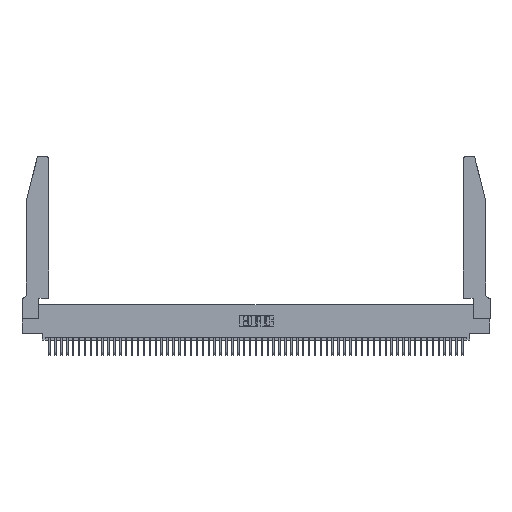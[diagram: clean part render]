
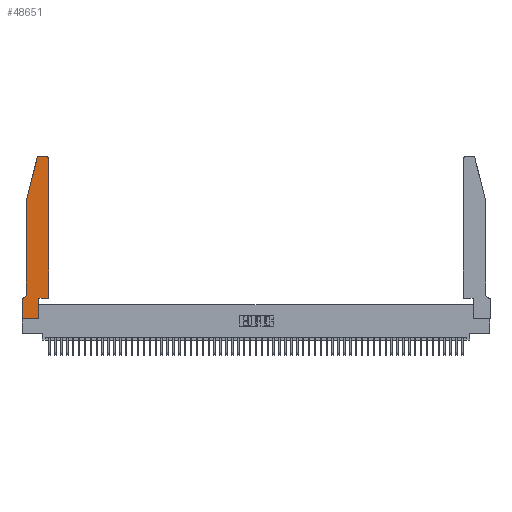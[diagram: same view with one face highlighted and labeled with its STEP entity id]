
A CAD part, top view. The second image highlights one B-rep face of the part: STEP entity #48651.
In plain terms, the highlighted planar face has unit normal (0, 0, 1).
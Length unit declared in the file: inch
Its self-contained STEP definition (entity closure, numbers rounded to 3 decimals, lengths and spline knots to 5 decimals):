
#319 = CARTESIAN_POINT ( 'NONE',  ( 0.0755, 2., 0.37 ) ) ;
#445 = AXIS2_PLACEMENT_3D ( 'NONE', #43484, #18274, #47694 ) ;
#1582 = EDGE_CURVE ( 'NONE', #11955, #36838, #24573, .T. ) ;
#1751 = CARTESIAN_POINT ( 'NONE',  ( 0.0055, 0.42, 0.37 ) ) ;
#1983 = CARTESIAN_POINT ( 'NONE',  ( 0., 0.35, 0.37 ) ) ;
#2160 = VECTOR ( 'NONE', #12118, 39.37008 ) ;
#3042 = CARTESIAN_POINT ( 'NONE',  ( 0.284, 2.75, 0.37 ) ) ;
#3897 = ORIENTED_EDGE ( 'NONE', *, *, #4796, .T. ) ;
#4695 = EDGE_CURVE ( 'NONE', #5324, #38068, #33540, .T. ) ;
#4796 = EDGE_CURVE ( 'NONE', #36075, #14396, #26893, .T. ) ;
#5324 = VERTEX_POINT ( 'NONE', #27573 ) ;
#6003 = DIRECTION ( 'NONE',  ( -1., 0., 0. ) ) ;
#6811 = ORIENTED_EDGE ( 'NONE', *, *, #1582, .T. ) ;
#7475 = CARTESIAN_POINT ( 'NONE',  ( 0.2865, 0.35, 0.37 ) ) ;
#7748 = EDGE_CURVE ( 'NONE', #14396, #22877, #35192, .T. ) ;
#8241 = EDGE_CURVE ( 'NONE', #36838, #21234, #42380, .T. ) ;
#8621 = VECTOR ( 'NONE', #40121, 39.37008 ) ;
#8830 = DIRECTION ( 'NONE',  ( 1., 0., 0. ) ) ;
#9283 = DIRECTION ( 'NONE',  ( -1., 0., 0. ) ) ;
#9639 = CARTESIAN_POINT ( 'NONE',  ( 0.2865, 0.35, 0.37 ) ) ;
#10487 = DIRECTION ( 'NONE',  ( 0., 0., 1. ) ) ;
#10995 = EDGE_CURVE ( 'NONE', #21234, #36075, #44745, .T. ) ;
#11955 = VERTEX_POINT ( 'NONE', #27336 ) ;
#12118 = DIRECTION ( 'NONE',  ( 0., -1., 0. ) ) ;
#13052 = CARTESIAN_POINT ( 'NONE',  ( 0.4505, 0.35, 0.37 ) ) ;
#14396 = VERTEX_POINT ( 'NONE', #27456 ) ;
#15655 = CARTESIAN_POINT ( 'NONE',  ( 0., 0., 0.37 ) ) ;
#16152 = VECTOR ( 'NONE', #9283, 39.37008 ) ;
#16214 = CARTESIAN_POINT ( 'NONE',  ( 0., 0., 0.37 ) ) ;
#17419 = ORIENTED_EDGE ( 'NONE', *, *, #7748, .T. ) ;
#18274 = DIRECTION ( 'NONE',  ( 0., 0., 1. ) ) ;
#18337 = VECTOR ( 'NONE', #19895, 39.37008 ) ;
#18453 = ORIENTED_EDGE ( 'NONE', *, *, #51909, .T. ) ;
#18457 = EDGE_CURVE ( 'NONE', #36590, #21401, #35798, .T. ) ;
#18555 = ORIENTED_EDGE ( 'NONE', *, *, #10995, .T. ) ;
#19895 = DIRECTION ( 'NONE',  ( 0., 1., 0. ) ) ;
#20871 = CARTESIAN_POINT ( 'NONE',  ( 0.0755, 0.42, 0.37 ) ) ;
#21234 = VERTEX_POINT ( 'NONE', #7475 ) ;
#21401 = VERTEX_POINT ( 'NONE', #20871 ) ;
#21773 = CARTESIAN_POINT ( 'NONE',  ( 0.2605, 2.75, 0.37 ) ) ;
#22257 = CIRCLE ( 'NONE', #445, 0.03 ) ;
#22319 = VECTOR ( 'NONE', #8830, 39.37008 ) ;
#22877 = VERTEX_POINT ( 'NONE', #31400 ) ;
#23267 = DIRECTION ( 'NONE',  ( 0., 0., 1. ) ) ;
#24428 = CIRCLE ( 'NONE', #27791, 0.07 ) ;
#24573 = LINE ( 'NONE', #16214, #49570 ) ;
#26893 = LINE ( 'NONE', #36698, #18337 ) ;
#27336 = CARTESIAN_POINT ( 'NONE',  ( 0., 0., 0.37 ) ) ;
#27456 = CARTESIAN_POINT ( 'NONE',  ( 0.4505, 2.72, 0.37 ) ) ;
#27573 = CARTESIAN_POINT ( 'NONE',  ( 0.0055, 0.35, 0.37 ) ) ;
#27791 = AXIS2_PLACEMENT_3D ( 'NONE', #1751, #31198, #6003 ) ;
#27898 = EDGE_CURVE ( 'NONE', #38068, #11955, #40880, .T. ) ;
#28631 = ORIENTED_EDGE ( 'NONE', *, *, #18457, .T. ) ;
#30777 = ORIENTED_EDGE ( 'NONE', *, *, #34444, .T. ) ;
#31198 = DIRECTION ( 'NONE',  ( 0., 0., -1. ) ) ;
#31400 = CARTESIAN_POINT ( 'NONE',  ( 0.4205, 2.75, 0.37 ) ) ;
#32064 = CARTESIAN_POINT ( 'NONE',  ( 0.0755, 0.35, 0.37 ) ) ;
#32835 = VERTEX_POINT ( 'NONE', #3042 ) ;
#33135 = CARTESIAN_POINT ( 'NONE',  ( 0.0755, 2., 0.37 ) ) ;
#33389 = ORIENTED_EDGE ( 'NONE', *, *, #49788, .T. ) ;
#33540 = LINE ( 'NONE', #32064, #51865 ) ;
#33965 = AXIS2_PLACEMENT_3D ( 'NONE', #48462, #23267, #52670 ) ;
#34058 = DIRECTION ( 'NONE',  ( -0.239, -0.971, 0. ) ) ;
#34444 = EDGE_CURVE ( 'NONE', #21401, #5324, #24428, .T. ) ;
#35192 = CIRCLE ( 'NONE', #33965, 0.03 ) ;
#35705 = CARTESIAN_POINT ( 'NONE',  ( 0.0755, 2., 0.37 ) ) ;
#35798 = LINE ( 'NONE', #33135, #2160 ) ;
#36075 = VERTEX_POINT ( 'NONE', #48189 ) ;
#36590 = VERTEX_POINT ( 'NONE', #35705 ) ;
#36698 = CARTESIAN_POINT ( 'NONE',  ( 0.4505, 0.35, 0.37 ) ) ;
#36838 = VERTEX_POINT ( 'NONE', #49974 ) ;
#38068 = VERTEX_POINT ( 'NONE', #46728 ) ;
#38545 = AXIS2_PLACEMENT_3D ( 'NONE', #1983, #10487, #39914 ) ;
#39551 = PLANE ( 'NONE',  #38545 ) ;
#39914 = DIRECTION ( 'NONE',  ( 1., 0., 0. ) ) ;
#40121 = DIRECTION ( 'NONE',  ( 0., -1., 0. ) ) ;
#40672 = EDGE_LOOP ( 'NONE', ( #46254, #33389, #18453, #28631, #30777, #40823, #45233, #6811, #53224, #18555, #3897, #17419 ) ) ;
#40823 = ORIENTED_EDGE ( 'NONE', *, *, #4695, .T. ) ;
#40880 = LINE ( 'NONE', #15655, #8621 ) ;
#42380 = LINE ( 'NONE', #9639, #43663 ) ;
#43484 = CARTESIAN_POINT ( 'NONE',  ( 0.284, 2.72, 0.37 ) ) ;
#43663 = VECTOR ( 'NONE', #47333, 39.37008 ) ;
#44045 = CARTESIAN_POINT ( 'NONE',  ( 0.25487, 2.72718, 0.37 ) ) ;
#44129 = FACE_OUTER_BOUND ( 'NONE', #40672, .T. ) ;
#44745 = LINE ( 'NONE', #13052, #22319 ) ;
#45233 = ORIENTED_EDGE ( 'NONE', *, *, #27898, .T. ) ;
#45664 = DIRECTION ( 'NONE',  ( 1., 0., 0. ) ) ;
#45733 = VECTOR ( 'NONE', #34058, 39.37008 ) ;
#46254 = ORIENTED_EDGE ( 'NONE', *, *, #51373, .T. ) ;
#46728 = CARTESIAN_POINT ( 'NONE',  ( 0., 0.35, 0.37 ) ) ;
#47025 = LINE ( 'NONE', #319, #45733 ) ;
#47333 = DIRECTION ( 'NONE',  ( 0., 1., 0. ) ) ;
#47694 = DIRECTION ( 'NONE',  ( 1., 0., 0. ) ) ;
#48189 = CARTESIAN_POINT ( 'NONE',  ( 0.4505, 0.35, 0.37 ) ) ;
#48462 = CARTESIAN_POINT ( 'NONE',  ( 0.4205, 2.72, 0.37 ) ) ;
#48651 = ADVANCED_FACE ( 'NONE', ( #44129 ), #39551, .T. ) ;
#49570 = VECTOR ( 'NONE', #45664, 39.37008 ) ;
#49713 = LINE ( 'NONE', #21773, #16152 ) ;
#49788 = EDGE_CURVE ( 'NONE', #32835, #52789, #22257, .T. ) ;
#49974 = CARTESIAN_POINT ( 'NONE',  ( 0.2865, 0., 0.37 ) ) ;
#51373 = EDGE_CURVE ( 'NONE', #22877, #32835, #49713, .T. ) ;
#51865 = VECTOR ( 'NONE', #52958, 39.37008 ) ;
#51909 = EDGE_CURVE ( 'NONE', #52789, #36590, #47025, .T. ) ;
#52670 = DIRECTION ( 'NONE',  ( 1., 0., 0. ) ) ;
#52789 = VERTEX_POINT ( 'NONE', #44045 ) ;
#52958 = DIRECTION ( 'NONE',  ( -1., 0., 0. ) ) ;
#53224 = ORIENTED_EDGE ( 'NONE', *, *, #8241, .T. ) ;
